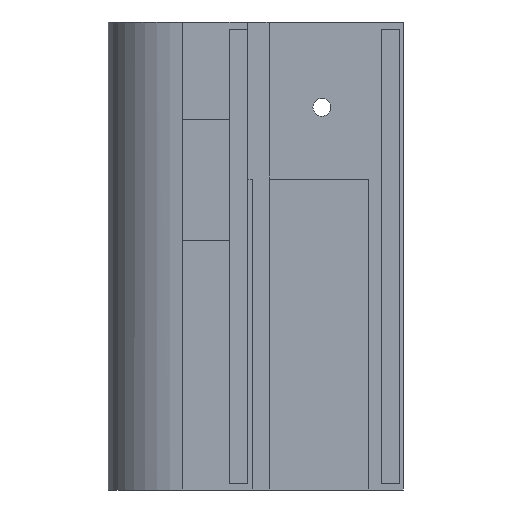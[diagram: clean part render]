
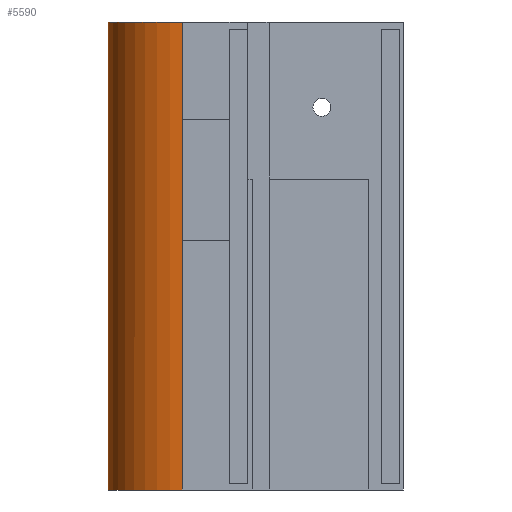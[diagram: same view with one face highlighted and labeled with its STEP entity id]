
A CAD part, left-side view. The second image highlights one B-rep face of the part: STEP entity #5590.
In plain terms, the highlighted cylindrical face has radius 13 mm (diameter 26 mm), a partial arc.
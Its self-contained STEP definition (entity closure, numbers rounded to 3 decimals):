
#1217 = PLANE('',#1218);
#1218 = AXIS2_PLACEMENT_3D('',#1219,#1220,#1221);
#1219 = CARTESIAN_POINT('',(-13.398,41.611,76.189));
#1220 = DIRECTION('',(0.,0.,1.));
#1221 = DIRECTION('',(1.,0.,0.));
#2782 = VERTEX_POINT('',#2783);
#2783 = CARTESIAN_POINT('',(-12.982,25.692,76.189));
#2798 = PLANE('',#2799);
#2799 = AXIS2_PLACEMENT_3D('',#2800,#2801,#2802);
#2800 = CARTESIAN_POINT('',(-18.356,47.561,-1.));
#2801 = DIRECTION('',(0.971,0.239,0.));
#2802 = DIRECTION('',(0.239,-0.971,0.));
#3210 = VERTEX_POINT('',#3211);
#3211 = CARTESIAN_POINT('',(12.986,25.605,76.189));
#3224 = PLANE('',#3225);
#3225 = AXIS2_PLACEMENT_3D('',#3226,#3227,#3228);
#3226 = CARTESIAN_POINT('',(12.986,25.605,-1.));
#3227 = DIRECTION('',(-0.989,0.145,0.));
#3228 = DIRECTION('',(0.145,0.989,0.));
#3235 = EDGE_CURVE('',#2782,#3210,#3236,.T.);
#3236 = SURFACE_CURVE('',#3237,(#3242,#3253),.PCURVE_S1.);
#3237 = CIRCLE('',#3238,13.);
#3238 = AXIS2_PLACEMENT_3D('',#3239,#3240,#3241);
#3239 = CARTESIAN_POINT('',(0.,25.,76.189));
#3240 = DIRECTION('',(0.,0.,-1.));
#3241 = DIRECTION('',(1.,0.,0.));
#3242 = PCURVE('',#1217,#3243);
#3243 = DEFINITIONAL_REPRESENTATION('',(#3244),#3252);
#3244 = ( BOUNDED_CURVE() B_SPLINE_CURVE(2,(#3245,#3246,#3247,#3248,
#3249,#3250,#3251),.UNSPECIFIED.,.T.,.F.) B_SPLINE_CURVE_WITH_KNOTS((1,2
    ,2,2,2,1),(-2.094,0.,2.094,4.189,
6.283,8.378),.UNSPECIFIED.) CURVE() 
GEOMETRIC_REPRESENTATION_ITEM() RATIONAL_B_SPLINE_CURVE((1.,0.5,1.,0.5,
1.,0.5,1.)) REPRESENTATION_ITEM('') );
#3245 = CARTESIAN_POINT('',(26.398,-16.611));
#3246 = CARTESIAN_POINT('',(26.398,-39.127));
#3247 = CARTESIAN_POINT('',(6.898,-27.869));
#3248 = CARTESIAN_POINT('',(-12.602,-16.611));
#3249 = CARTESIAN_POINT('',(6.898,-5.352));
#3250 = CARTESIAN_POINT('',(26.398,5.906));
#3251 = CARTESIAN_POINT('',(26.398,-16.611));
#3252 = ( GEOMETRIC_REPRESENTATION_CONTEXT(2) 
PARAMETRIC_REPRESENTATION_CONTEXT() REPRESENTATION_CONTEXT('2D SPACE',''
  ) );
#3253 = PCURVE('',#3254,#3259);
#3254 = CYLINDRICAL_SURFACE('',#3255,13.);
#3255 = AXIS2_PLACEMENT_3D('',#3256,#3257,#3258);
#3256 = CARTESIAN_POINT('',(0.,25.,-1.));
#3257 = DIRECTION('',(0.,0.,-1.));
#3258 = DIRECTION('',(1.,0.,0.));
#3259 = DEFINITIONAL_REPRESENTATION('',(#3260),#3264);
#3260 = LINE('',#3261,#3262);
#3261 = CARTESIAN_POINT('',(0.,-77.189));
#3262 = VECTOR('',#3263,1.);
#3263 = DIRECTION('',(1.,0.));
#3264 = ( GEOMETRIC_REPRESENTATION_CONTEXT(2) 
PARAMETRIC_REPRESENTATION_CONTEXT() REPRESENTATION_CONTEXT('2D SPACE',''
  ) );
#5471 = VERTEX_POINT('',#5472);
#5472 = CARTESIAN_POINT('',(-12.982,25.692,-1.));
#5486 = PLANE('',#5487);
#5487 = AXIS2_PLACEMENT_3D('',#5488,#5489,#5490);
#5488 = CARTESIAN_POINT('',(-13.,-5.,-1.));
#5489 = DIRECTION('',(0.,0.,-1.));
#5490 = DIRECTION('',(-1.,0.,0.));
#5570 = EDGE_CURVE('',#5471,#2782,#5571,.T.);
#5571 = SURFACE_CURVE('',#5572,(#5576,#5583),.PCURVE_S1.);
#5572 = LINE('',#5573,#5574);
#5573 = CARTESIAN_POINT('',(-12.982,25.692,-1.));
#5574 = VECTOR('',#5575,1.);
#5575 = DIRECTION('',(0.,0.,1.));
#5576 = PCURVE('',#2798,#5577);
#5577 = DEFINITIONAL_REPRESENTATION('',(#5578),#5582);
#5578 = LINE('',#5579,#5580);
#5579 = CARTESIAN_POINT('',(22.52,0.));
#5580 = VECTOR('',#5581,1.);
#5581 = DIRECTION('',(0.,-1.));
#5582 = ( GEOMETRIC_REPRESENTATION_CONTEXT(2) 
PARAMETRIC_REPRESENTATION_CONTEXT() REPRESENTATION_CONTEXT('2D SPACE',''
  ) );
#5583 = PCURVE('',#3254,#5584);
#5584 = DEFINITIONAL_REPRESENTATION('',(#5585),#5589);
#5585 = LINE('',#5586,#5587);
#5586 = CARTESIAN_POINT('',(3.195,0.));
#5587 = VECTOR('',#5588,1.);
#5588 = DIRECTION('',(0.,-1.));
#5589 = ( GEOMETRIC_REPRESENTATION_CONTEXT(2) 
PARAMETRIC_REPRESENTATION_CONTEXT() REPRESENTATION_CONTEXT('2D SPACE',''
  ) );
#5590 = ADVANCED_FACE('',(#5591),#3254,.T.);
#5591 = FACE_BOUND('',#5592,.T.);
#5592 = EDGE_LOOP('',(#5593,#5617,#5618,#5619,#5642,#5671));
#5593 = ORIENTED_EDGE('',*,*,#5594,.F.);
#5594 = EDGE_CURVE('',#5471,#5595,#5597,.T.);
#5595 = VERTEX_POINT('',#5596);
#5596 = CARTESIAN_POINT('',(-11.,31.928,-1.));
#5597 = SURFACE_CURVE('',#5598,(#5603,#5610),.PCURVE_S1.);
#5598 = CIRCLE('',#5599,13.);
#5599 = AXIS2_PLACEMENT_3D('',#5600,#5601,#5602);
#5600 = CARTESIAN_POINT('',(0.,25.,-1.));
#5601 = DIRECTION('',(0.,0.,-1.));
#5602 = DIRECTION('',(1.,0.,0.));
#5603 = PCURVE('',#3254,#5604);
#5604 = DEFINITIONAL_REPRESENTATION('',(#5605),#5609);
#5605 = LINE('',#5606,#5607);
#5606 = CARTESIAN_POINT('',(0.,0.));
#5607 = VECTOR('',#5608,1.);
#5608 = DIRECTION('',(1.,0.));
#5609 = ( GEOMETRIC_REPRESENTATION_CONTEXT(2) 
PARAMETRIC_REPRESENTATION_CONTEXT() REPRESENTATION_CONTEXT('2D SPACE',''
  ) );
#5610 = PCURVE('',#5486,#5611);
#5611 = DEFINITIONAL_REPRESENTATION('',(#5612),#5616);
#5612 = CIRCLE('',#5613,13.);
#5613 = AXIS2_PLACEMENT_2D('',#5614,#5615);
#5614 = CARTESIAN_POINT('',(-13.,30.));
#5615 = DIRECTION('',(-1.,0.));
#5616 = ( GEOMETRIC_REPRESENTATION_CONTEXT(2) 
PARAMETRIC_REPRESENTATION_CONTEXT() REPRESENTATION_CONTEXT('2D SPACE',''
  ) );
#5617 = ORIENTED_EDGE('',*,*,#5570,.T.);
#5618 = ORIENTED_EDGE('',*,*,#3235,.T.);
#5619 = ORIENTED_EDGE('',*,*,#5620,.F.);
#5620 = EDGE_CURVE('',#5621,#3210,#5623,.T.);
#5621 = VERTEX_POINT('',#5622);
#5622 = CARTESIAN_POINT('',(12.986,25.605,-1.));
#5623 = SURFACE_CURVE('',#5624,(#5628,#5635),.PCURVE_S1.);
#5624 = LINE('',#5625,#5626);
#5625 = CARTESIAN_POINT('',(12.986,25.605,-1.));
#5626 = VECTOR('',#5627,1.);
#5627 = DIRECTION('',(0.,0.,1.));
#5628 = PCURVE('',#3254,#5629);
#5629 = DEFINITIONAL_REPRESENTATION('',(#5630),#5634);
#5630 = LINE('',#5631,#5632);
#5631 = CARTESIAN_POINT('',(6.237,0.));
#5632 = VECTOR('',#5633,1.);
#5633 = DIRECTION('',(0.,-1.));
#5634 = ( GEOMETRIC_REPRESENTATION_CONTEXT(2) 
PARAMETRIC_REPRESENTATION_CONTEXT() REPRESENTATION_CONTEXT('2D SPACE',''
  ) );
#5635 = PCURVE('',#3224,#5636);
#5636 = DEFINITIONAL_REPRESENTATION('',(#5637),#5641);
#5637 = LINE('',#5638,#5639);
#5638 = CARTESIAN_POINT('',(0.,0.));
#5639 = VECTOR('',#5640,1.);
#5640 = DIRECTION('',(0.,-1.));
#5641 = ( GEOMETRIC_REPRESENTATION_CONTEXT(2) 
PARAMETRIC_REPRESENTATION_CONTEXT() REPRESENTATION_CONTEXT('2D SPACE',''
  ) );
#5642 = ORIENTED_EDGE('',*,*,#5643,.F.);
#5643 = EDGE_CURVE('',#5644,#5621,#5646,.T.);
#5644 = VERTEX_POINT('',#5645);
#5645 = CARTESIAN_POINT('',(11.,31.928,-1.));
#5646 = SURFACE_CURVE('',#5647,(#5652,#5659),.PCURVE_S1.);
#5647 = CIRCLE('',#5648,13.);
#5648 = AXIS2_PLACEMENT_3D('',#5649,#5650,#5651);
#5649 = CARTESIAN_POINT('',(0.,25.,-1.));
#5650 = DIRECTION('',(0.,0.,-1.));
#5651 = DIRECTION('',(1.,0.,0.));
#5652 = PCURVE('',#3254,#5653);
#5653 = DEFINITIONAL_REPRESENTATION('',(#5654),#5658);
#5654 = LINE('',#5655,#5656);
#5655 = CARTESIAN_POINT('',(0.,0.));
#5656 = VECTOR('',#5657,1.);
#5657 = DIRECTION('',(1.,0.));
#5658 = ( GEOMETRIC_REPRESENTATION_CONTEXT(2) 
PARAMETRIC_REPRESENTATION_CONTEXT() REPRESENTATION_CONTEXT('2D SPACE',''
  ) );
#5659 = PCURVE('',#5660,#5665);
#5660 = PLANE('',#5661);
#5661 = AXIS2_PLACEMENT_3D('',#5662,#5663,#5664);
#5662 = CARTESIAN_POINT('',(-13.,-5.,-1.));
#5663 = DIRECTION('',(0.,0.,-1.));
#5664 = DIRECTION('',(-1.,0.,0.));
#5665 = DEFINITIONAL_REPRESENTATION('',(#5666),#5670);
#5666 = CIRCLE('',#5667,13.);
#5667 = AXIS2_PLACEMENT_2D('',#5668,#5669);
#5668 = CARTESIAN_POINT('',(-13.,30.));
#5669 = DIRECTION('',(-1.,0.));
#5670 = ( GEOMETRIC_REPRESENTATION_CONTEXT(2) 
PARAMETRIC_REPRESENTATION_CONTEXT() REPRESENTATION_CONTEXT('2D SPACE',''
  ) );
#5671 = ORIENTED_EDGE('',*,*,#5672,.F.);
#5672 = EDGE_CURVE('',#5595,#5644,#5673,.T.);
#5673 = SURFACE_CURVE('',#5674,(#5679,#5686),.PCURVE_S1.);
#5674 = CIRCLE('',#5675,13.);
#5675 = AXIS2_PLACEMENT_3D('',#5676,#5677,#5678);
#5676 = CARTESIAN_POINT('',(0.,25.,-1.));
#5677 = DIRECTION('',(0.,0.,-1.));
#5678 = DIRECTION('',(1.,0.,0.));
#5679 = PCURVE('',#3254,#5680);
#5680 = DEFINITIONAL_REPRESENTATION('',(#5681),#5685);
#5681 = LINE('',#5682,#5683);
#5682 = CARTESIAN_POINT('',(0.,0.));
#5683 = VECTOR('',#5684,1.);
#5684 = DIRECTION('',(1.,0.));
#5685 = ( GEOMETRIC_REPRESENTATION_CONTEXT(2) 
PARAMETRIC_REPRESENTATION_CONTEXT() REPRESENTATION_CONTEXT('2D SPACE',''
  ) );
#5686 = PCURVE('',#5687,#5692);
#5687 = PLANE('',#5688);
#5688 = AXIS2_PLACEMENT_3D('',#5689,#5690,#5691);
#5689 = CARTESIAN_POINT('',(-13.,-5.,-1.));
#5690 = DIRECTION('',(0.,0.,-1.));
#5691 = DIRECTION('',(-1.,0.,0.));
#5692 = DEFINITIONAL_REPRESENTATION('',(#5693),#5697);
#5693 = CIRCLE('',#5694,13.);
#5694 = AXIS2_PLACEMENT_2D('',#5695,#5696);
#5695 = CARTESIAN_POINT('',(-13.,30.));
#5696 = DIRECTION('',(-1.,0.));
#5697 = ( GEOMETRIC_REPRESENTATION_CONTEXT(2) 
PARAMETRIC_REPRESENTATION_CONTEXT() REPRESENTATION_CONTEXT('2D SPACE',''
  ) );
